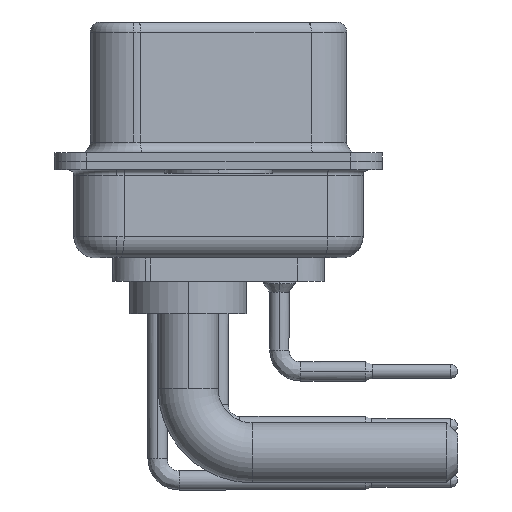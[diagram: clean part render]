
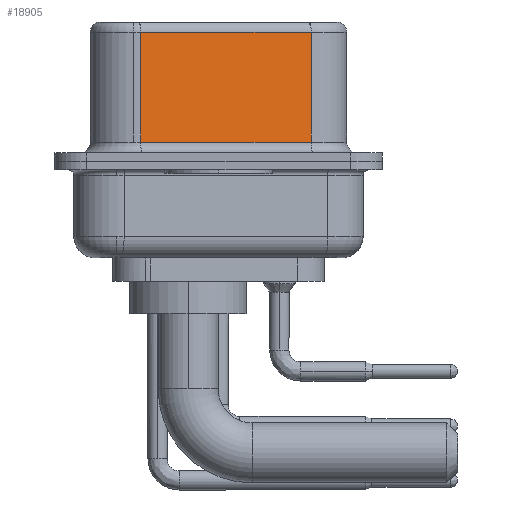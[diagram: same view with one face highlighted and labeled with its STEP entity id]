
A CAD part, left-side view. The second image highlights one B-rep face of the part: STEP entity #18905.
In plain terms, the highlighted planar face has unit normal (-0.985, -0.174, 0).
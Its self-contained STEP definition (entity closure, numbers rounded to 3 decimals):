
#389 = CARTESIAN_POINT ( 'NONE',  ( 5.132, -4.322, 0.9 ) ) ;
#1691 = PLANE ( 'NONE',  #14827 ) ;
#2010 = LINE ( 'NONE', #21715, #29834 ) ;
#3324 = CARTESIAN_POINT ( 'NONE',  ( 5.132, -4.322, 6.02 ) ) ;
#3879 = ORIENTED_EDGE ( 'NONE', *, *, #15693, .T. ) ;
#6790 = CARTESIAN_POINT ( 'NONE',  ( 5.132, -4.322, 6.52 ) ) ;
#8818 = EDGE_CURVE ( 'NONE', #28867, #12493, #19323, .T. ) ;
#10909 = LINE ( 'NONE', #24006, #11589 ) ;
#10947 = CARTESIAN_POINT ( 'NONE',  ( 3.73, 3.628, 0.9 ) ) ;
#11589 = VECTOR ( 'NONE', #23533, 1000. ) ;
#11867 = CARTESIAN_POINT ( 'NONE',  ( 3.73, 3.628, 6.02 ) ) ;
#12493 = VERTEX_POINT ( 'NONE', #389 ) ;
#14010 = DIRECTION ( 'NONE',  ( -0.174, 0.985, 0. ) ) ;
#14816 = ORIENTED_EDGE ( 'NONE', *, *, #8818, .T. ) ;
#14827 = AXIS2_PLACEMENT_3D ( 'NONE', #6790, #16619, #14010 ) ;
#15693 = EDGE_CURVE ( 'NONE', #30737, #28867, #10909, .T. ) ;
#16313 = DIRECTION ( 'NONE',  ( -0.174, 0.985, 0. ) ) ;
#16594 = VECTOR ( 'NONE', #20900, 1000. ) ;
#16619 = DIRECTION ( 'NONE',  ( 0.985, 0.174, 0. ) ) ;
#18905 = ADVANCED_FACE ( 'NONE', ( #25114 ), #1691, .F. ) ;
#19168 = CARTESIAN_POINT ( 'NONE',  ( 5.132, -4.322, 0.9 ) ) ;
#19323 = LINE ( 'NONE', #19168, #31966 ) ;
#20900 = DIRECTION ( 'NONE',  ( 0., 0., -1. ) ) ;
#21489 = DIRECTION ( 'NONE',  ( 0.174, -0.985, 0. ) ) ;
#21715 = CARTESIAN_POINT ( 'NONE',  ( 5.132, -4.322, 6.02 ) ) ;
#23533 = DIRECTION ( 'NONE',  ( 0., 0., -1. ) ) ;
#23604 = EDGE_LOOP ( 'NONE', ( #27019, #25158, #3879, #14816 ) ) ;
#23961 = EDGE_CURVE ( 'NONE', #24612, #12493, #27966, .T. ) ;
#24006 = CARTESIAN_POINT ( 'NONE',  ( 3.73, 3.628, 6.52 ) ) ;
#24612 = VERTEX_POINT ( 'NONE', #3324 ) ;
#25114 = FACE_OUTER_BOUND ( 'NONE', #23604, .T. ) ;
#25158 = ORIENTED_EDGE ( 'NONE', *, *, #31893, .T. ) ;
#27019 = ORIENTED_EDGE ( 'NONE', *, *, #23961, .F. ) ;
#27966 = LINE ( 'NONE', #31056, #16594 ) ;
#28867 = VERTEX_POINT ( 'NONE', #10947 ) ;
#29834 = VECTOR ( 'NONE', #16313, 1000. ) ;
#30737 = VERTEX_POINT ( 'NONE', #11867 ) ;
#31056 = CARTESIAN_POINT ( 'NONE',  ( 5.132, -4.322, 6.52 ) ) ;
#31893 = EDGE_CURVE ( 'NONE', #24612, #30737, #2010, .T. ) ;
#31966 = VECTOR ( 'NONE', #21489, 1000. ) ;
